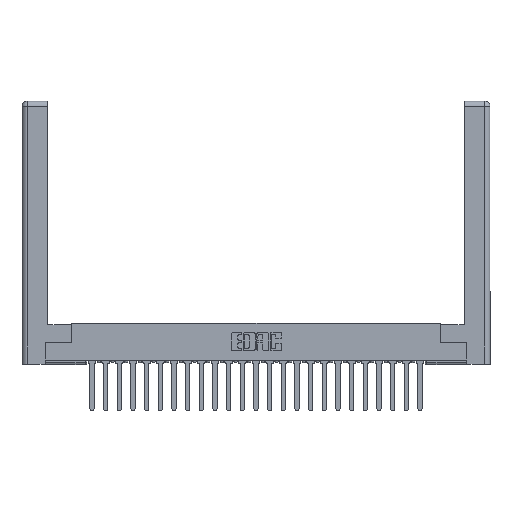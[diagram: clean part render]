
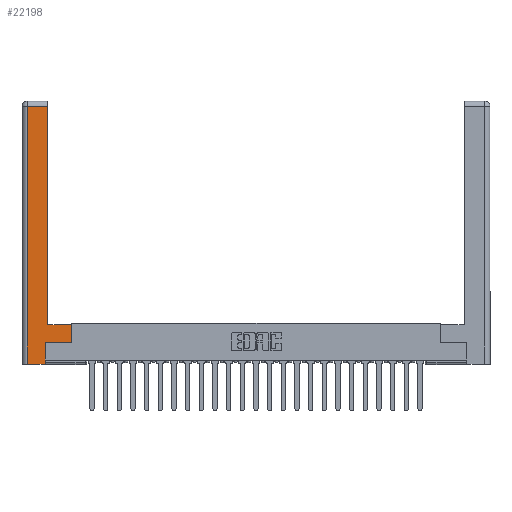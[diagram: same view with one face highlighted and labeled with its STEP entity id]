
A CAD part, top view. The second image highlights one B-rep face of the part: STEP entity #22198.
In plain terms, the highlighted planar face has unit normal (0, 0, 1).
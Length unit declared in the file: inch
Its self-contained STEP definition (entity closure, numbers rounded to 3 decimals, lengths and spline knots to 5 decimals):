
#1030 = LINE ( 'NONE', #5286, #7546 ) ;
#1313 = ORIENTED_EDGE ( 'NONE', *, *, #3478, .T. ) ;
#1476 = DIRECTION ( 'NONE',  ( -1., 0., 0. ) ) ;
#1763 = DIRECTION ( 'NONE',  ( -1., 0., 0. ) ) ;
#1868 = CARTESIAN_POINT ( 'NONE',  ( 0.565, 0.245, 0. ) ) ;
#3077 = CARTESIAN_POINT ( 'NONE',  ( 0.0615, 0., 0. ) ) ;
#3435 = DIRECTION ( 'NONE',  ( 1., 0., 0. ) ) ;
#3478 = EDGE_CURVE ( 'NONE', #11951, #21249, #21823, .T. ) ;
#3672 = VECTOR ( 'NONE', #1476, 39.37008 ) ;
#3914 = VECTOR ( 'NONE', #21050, 39.37008 ) ;
#4080 = ORIENTED_EDGE ( 'NONE', *, *, #23933, .T. ) ;
#4330 = CARTESIAN_POINT ( 'NONE',  ( 0.295, 3., 0. ) ) ;
#5286 = CARTESIAN_POINT ( 'NONE',  ( 0.0615, 0., 0. ) ) ;
#5444 = VECTOR ( 'NONE', #1763, 39.37008 ) ;
#5752 = VERTEX_POINT ( 'NONE', #11188 ) ;
#5817 = CARTESIAN_POINT ( 'NONE',  ( 0.295, 0.45, 0. ) ) ;
#5836 = LINE ( 'NONE', #11751, #21772 ) ;
#6523 = VERTEX_POINT ( 'NONE', #16947 ) ;
#6925 = AXIS2_PLACEMENT_3D ( 'NONE', #9218, #25629, #13245 ) ;
#6943 = PLANE ( 'NONE',  #6925 ) ;
#7320 = VECTOR ( 'NONE', #15906, 39.37008 ) ;
#7497 = ORIENTED_EDGE ( 'NONE', *, *, #16123, .T. ) ;
#7539 = FACE_OUTER_BOUND ( 'NONE', #12309, .T. ) ;
#7546 = VECTOR ( 'NONE', #25955, 39.37008 ) ;
#8356 = DIRECTION ( 'NONE',  ( 0., 1., 0. ) ) ;
#9218 = CARTESIAN_POINT ( 'NONE',  ( 0., 0., 0. ) ) ;
#9670 = LINE ( 'NONE', #26755, #5444 ) ;
#9837 = ORIENTED_EDGE ( 'NONE', *, *, #11608, .T. ) ;
#10314 = EDGE_CURVE ( 'NONE', #22860, #11951, #16118, .T. ) ;
#11188 = CARTESIAN_POINT ( 'NONE',  ( 0.295, 2.94, 0. ) ) ;
#11608 = EDGE_CURVE ( 'NONE', #21212, #5752, #24153, .T. ) ;
#11751 = CARTESIAN_POINT ( 'NONE',  ( 0.265, 0., 0. ) ) ;
#11951 = VERTEX_POINT ( 'NONE', #21524 ) ;
#12309 = EDGE_LOOP ( 'NONE', ( #9837, #13070, #16835, #7497, #17736, #1313, #4080, #15157 ) ) ;
#12387 = LINE ( 'NONE', #22723, #12698 ) ;
#12590 = EDGE_CURVE ( 'NONE', #20715, #21212, #20278, .T. ) ;
#12698 = VECTOR ( 'NONE', #8356, 39.37008 ) ;
#13070 = ORIENTED_EDGE ( 'NONE', *, *, #16918, .T. ) ;
#13227 = VERTEX_POINT ( 'NONE', #3077 ) ;
#13245 = DIRECTION ( 'NONE',  ( -1., 0., 0. ) ) ;
#15157 = ORIENTED_EDGE ( 'NONE', *, *, #12590, .T. ) ;
#15544 = CARTESIAN_POINT ( 'NONE',  ( 0.265, 0.245, 0. ) ) ;
#15906 = DIRECTION ( 'NONE',  ( 0., 1., 0. ) ) ;
#16118 = LINE ( 'NONE', #15544, #7320 ) ;
#16123 = EDGE_CURVE ( 'NONE', #13227, #22860, #5836, .T. ) ;
#16835 = ORIENTED_EDGE ( 'NONE', *, *, #22804, .T. ) ;
#16918 = EDGE_CURVE ( 'NONE', #5752, #6523, #9670, .T. ) ;
#16947 = CARTESIAN_POINT ( 'NONE',  ( 0.0615, 2.94, 0. ) ) ;
#17736 = ORIENTED_EDGE ( 'NONE', *, *, #10314, .T. ) ;
#18795 = DIRECTION ( 'NONE',  ( 0., 1., 0. ) ) ;
#18969 = CARTESIAN_POINT ( 'NONE',  ( 0.565, 0.245, 0. ) ) ;
#20278 = LINE ( 'NONE', #22125, #3672 ) ;
#20586 = VECTOR ( 'NONE', #18795, 39.37008 ) ;
#20715 = VERTEX_POINT ( 'NONE', #21087 ) ;
#21050 = DIRECTION ( 'NONE',  ( 1., 0., 0. ) ) ;
#21087 = CARTESIAN_POINT ( 'NONE',  ( 0.565, 0.45, 0. ) ) ;
#21212 = VERTEX_POINT ( 'NONE', #5817 ) ;
#21249 = VERTEX_POINT ( 'NONE', #1868 ) ;
#21524 = CARTESIAN_POINT ( 'NONE',  ( 0.265, 0.245, 0. ) ) ;
#21772 = VECTOR ( 'NONE', #3435, 39.37008 ) ;
#21823 = LINE ( 'NONE', #18969, #3914 ) ;
#22125 = CARTESIAN_POINT ( 'NONE',  ( 0.295, 0.45, 0. ) ) ;
#22198 = ADVANCED_FACE ( 'NONE', ( #7539 ), #6943, .F. ) ;
#22723 = CARTESIAN_POINT ( 'NONE',  ( 0.565, 0.45, 0. ) ) ;
#22804 = EDGE_CURVE ( 'NONE', #6523, #13227, #1030, .T. ) ;
#22860 = VERTEX_POINT ( 'NONE', #23641 ) ;
#23641 = CARTESIAN_POINT ( 'NONE',  ( 0.265, 0., 0. ) ) ;
#23933 = EDGE_CURVE ( 'NONE', #21249, #20715, #12387, .T. ) ;
#24153 = LINE ( 'NONE', #4330, #20586 ) ;
#25629 = DIRECTION ( 'NONE',  ( 0., 0., -1. ) ) ;
#25955 = DIRECTION ( 'NONE',  ( 0., -1., 0. ) ) ;
#26755 = CARTESIAN_POINT ( 'NONE',  ( 0.0615, 2.94, 0. ) ) ;
